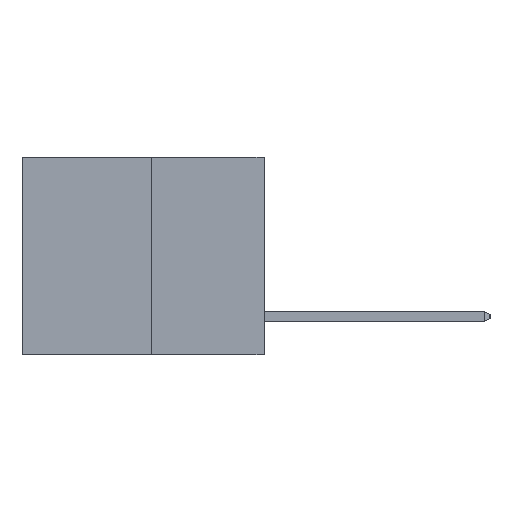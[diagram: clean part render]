
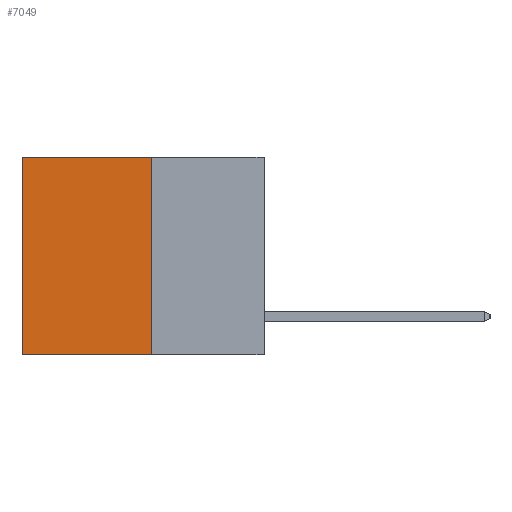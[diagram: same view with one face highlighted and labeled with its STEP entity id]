
A CAD part, left-side view. The second image highlights one B-rep face of the part: STEP entity #7049.
In plain terms, the highlighted planar face has unit normal (-1, 0, 0).
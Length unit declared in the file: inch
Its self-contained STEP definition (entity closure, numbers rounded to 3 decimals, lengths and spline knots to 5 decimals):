
#758 = DIRECTION ( 'NONE',  ( 1., 0., 0. ) ) ;
#819 = PLANE ( 'NONE',  #3158 ) ;
#909 = CARTESIAN_POINT ( 'NONE',  ( 0.3165, 0.28, -0.49 ) ) ;
#938 = DIRECTION ( 'NONE',  ( 0., 1., 0. ) ) ;
#2287 = VECTOR ( 'NONE', #938, 39.37008 ) ;
#2503 = VERTEX_POINT ( 'NONE', #15296 ) ;
#2768 = VERTEX_POINT ( 'NONE', #909 ) ;
#2908 = DIRECTION ( 'NONE',  ( 0., 1., 0. ) ) ;
#3068 = LINE ( 'NONE', #12596, #4805 ) ;
#3158 = AXIS2_PLACEMENT_3D ( 'NONE', #12142, #758, #4954 ) ;
#3186 = EDGE_CURVE ( 'NONE', #2768, #2503, #4611, .T. ) ;
#4244 = FACE_OUTER_BOUND ( 'NONE', #10758, .T. ) ;
#4347 = EDGE_CURVE ( 'NONE', #7012, #7118, #13608, .T. ) ;
#4611 = LINE ( 'NONE', #16635, #16587 ) ;
#4747 = VECTOR ( 'NONE', #7903, 39.37008 ) ;
#4805 = VECTOR ( 'NONE', #13768, 39.37008 ) ;
#4954 = DIRECTION ( 'NONE',  ( 0., 0., -1. ) ) ;
#7012 = VERTEX_POINT ( 'NONE', #16026 ) ;
#7049 = ADVANCED_FACE ( 'NONE', ( #4244 ), #819, .F. ) ;
#7118 = VERTEX_POINT ( 'NONE', #16573 ) ;
#7903 = DIRECTION ( 'NONE',  ( 0., 0., -1. ) ) ;
#9389 = ORIENTED_EDGE ( 'NONE', *, *, #10773, .T. ) ;
#10758 = EDGE_LOOP ( 'NONE', ( #9389, #15066, #11486, #16711 ) ) ;
#10773 = EDGE_CURVE ( 'NONE', #7118, #2503, #3068, .T. ) ;
#11486 = ORIENTED_EDGE ( 'NONE', *, *, #12519, .F. ) ;
#12142 = CARTESIAN_POINT ( 'NONE',  ( 0.3165, 0.28, -0.49 ) ) ;
#12519 = EDGE_CURVE ( 'NONE', #7012, #2768, #16922, .T. ) ;
#12596 = CARTESIAN_POINT ( 'NONE',  ( 0.3165, 0.6, -0.49 ) ) ;
#13418 = CARTESIAN_POINT ( 'NONE',  ( 0.3165, 0.28, 0. ) ) ;
#13608 = LINE ( 'NONE', #13418, #2287 ) ;
#13768 = DIRECTION ( 'NONE',  ( 0., 0., -1. ) ) ;
#14765 = CARTESIAN_POINT ( 'NONE',  ( 0.3165, 0.28, -0.49 ) ) ;
#15066 = ORIENTED_EDGE ( 'NONE', *, *, #3186, .F. ) ;
#15296 = CARTESIAN_POINT ( 'NONE',  ( 0.3165, 0.6, -0.49 ) ) ;
#16026 = CARTESIAN_POINT ( 'NONE',  ( 0.3165, 0.28, 0. ) ) ;
#16573 = CARTESIAN_POINT ( 'NONE',  ( 0.3165, 0.6, 0. ) ) ;
#16587 = VECTOR ( 'NONE', #2908, 39.37008 ) ;
#16635 = CARTESIAN_POINT ( 'NONE',  ( 0.3165, 0.28, -0.49 ) ) ;
#16711 = ORIENTED_EDGE ( 'NONE', *, *, #4347, .T. ) ;
#16922 = LINE ( 'NONE', #14765, #4747 ) ;
